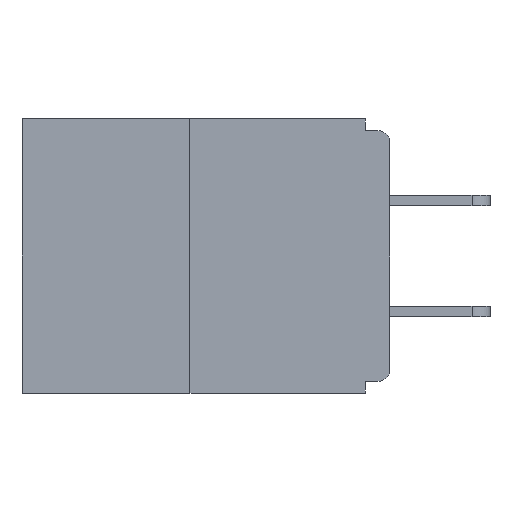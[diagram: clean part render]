
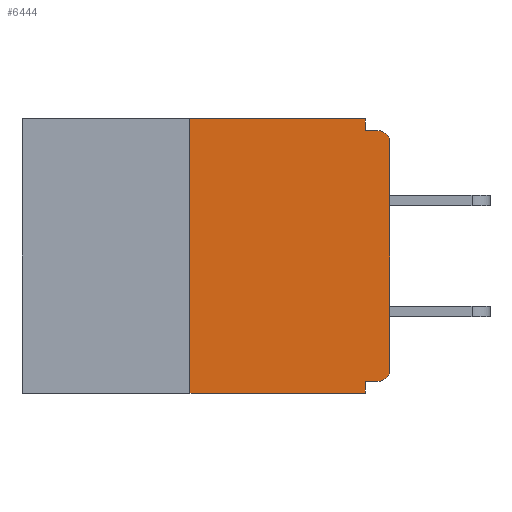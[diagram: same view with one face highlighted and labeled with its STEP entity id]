
A CAD part, left-side view. The second image highlights one B-rep face of the part: STEP entity #6444.
In plain terms, the highlighted planar face has unit normal (-1, 0, 0).
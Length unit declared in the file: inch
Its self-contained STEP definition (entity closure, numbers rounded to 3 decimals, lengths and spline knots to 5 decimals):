
#182 = VERTEX_POINT ( 'NONE', #7710 ) ;
#297 = ORIENTED_EDGE ( 'NONE', *, *, #10551, .T. ) ;
#424 = DIRECTION ( 'NONE',  ( 0., 1., 0. ) ) ;
#600 = ORIENTED_EDGE ( 'NONE', *, *, #10276, .T. ) ;
#846 = EDGE_CURVE ( 'NONE', #17180, #11150, #14406, .T. ) ;
#995 = LINE ( 'NONE', #12492, #16593 ) ;
#1286 = CARTESIAN_POINT ( 'NONE',  ( 0., 0.031, -0.015 ) ) ;
#1500 = CARTESIAN_POINT ( 'NONE',  ( 0., 0.031, -0.343 ) ) ;
#1552 = DIRECTION ( 'NONE',  ( 0., 0., 1. ) ) ;
#1807 = ORIENTED_EDGE ( 'NONE', *, *, #14363, .T. ) ;
#1910 = VECTOR ( 'NONE', #12389, 39.37008 ) ;
#2256 = CARTESIAN_POINT ( 'NONE',  ( 0., 0.031, -0.343 ) ) ;
#2279 = DIRECTION ( 'NONE',  ( 0., 0., -1. ) ) ;
#2557 = VECTOR ( 'NONE', #3654, 39.37008 ) ;
#3417 = ORIENTED_EDGE ( 'NONE', *, *, #14529, .F. ) ;
#3524 = LINE ( 'NONE', #6114, #14018 ) ;
#3570 = ORIENTED_EDGE ( 'NONE', *, *, #10451, .F. ) ;
#3654 = DIRECTION ( 'NONE',  ( 0., -1., 0. ) ) ;
#3727 = DIRECTION ( 'NONE',  ( 0., 0., 1. ) ) ;
#3900 = DIRECTION ( 'NONE',  ( 0., 0., -1. ) ) ;
#3932 = EDGE_CURVE ( 'NONE', #16206, #17180, #12841, .T. ) ;
#3948 = VERTEX_POINT ( 'NONE', #15938 ) ;
#3962 = PLANE ( 'NONE',  #10480 ) ;
#4166 = FACE_OUTER_BOUND ( 'NONE', #7609, .T. ) ;
#4472 = AXIS2_PLACEMENT_3D ( 'NONE', #9068, #15980, #2279 ) ;
#4695 = VERTEX_POINT ( 'NONE', #12079 ) ;
#5044 = CARTESIAN_POINT ( 'NONE',  ( 0., 0.25, 0. ) ) ;
#5382 = CARTESIAN_POINT ( 'NONE',  ( 0., 0.015, -0.328 ) ) ;
#5787 = EDGE_CURVE ( 'NONE', #13504, #9596, #6554, .T. ) ;
#6114 = CARTESIAN_POINT ( 'NONE',  ( 0., 0., -0.015 ) ) ;
#6289 = AXIS2_PLACEMENT_3D ( 'NONE', #17013, #10186, #7740 ) ;
#6444 = ADVANCED_FACE ( 'NONE', ( #4166 ), #3962, .F. ) ;
#6542 = VECTOR ( 'NONE', #424, 39.37008 ) ;
#6547 = ORIENTED_EDGE ( 'NONE', *, *, #5787, .T. ) ;
#6554 = LINE ( 'NONE', #6961, #10618 ) ;
#6961 = CARTESIAN_POINT ( 'NONE',  ( 0., 0.46, -0.343 ) ) ;
#6997 = CIRCLE ( 'NONE', #4472, 0.015 ) ;
#7045 = VECTOR ( 'NONE', #3727, 39.37008 ) ;
#7468 = LINE ( 'NONE', #5044, #7045 ) ;
#7609 = EDGE_LOOP ( 'NONE', ( #11813, #13123, #6547, #3417, #15741, #1807, #297, #600, #3570, #8094 ) ) ;
#7710 = CARTESIAN_POINT ( 'NONE',  ( 0., 0., -0.313 ) ) ;
#7727 = CIRCLE ( 'NONE', #6289, 0.015 ) ;
#7740 = DIRECTION ( 'NONE',  ( 0., 0., -1. ) ) ;
#8094 = ORIENTED_EDGE ( 'NONE', *, *, #846, .F. ) ;
#8153 = VERTEX_POINT ( 'NONE', #5382 ) ;
#8978 = CARTESIAN_POINT ( 'NONE',  ( 0., 0., -0.03 ) ) ;
#9068 = CARTESIAN_POINT ( 'NONE',  ( 0., 0.015, -0.03 ) ) ;
#9596 = VERTEX_POINT ( 'NONE', #2256 ) ;
#9600 = DIRECTION ( 'NONE',  ( 0., 0., -1. ) ) ;
#9666 = CARTESIAN_POINT ( 'NONE',  ( 0., 0.25, 0. ) ) ;
#10186 = DIRECTION ( 'NONE',  ( -1., 0., 0. ) ) ;
#10276 = EDGE_CURVE ( 'NONE', #13741, #3948, #6997, .T. ) ;
#10451 = EDGE_CURVE ( 'NONE', #11150, #3948, #3524, .T. ) ;
#10480 = AXIS2_PLACEMENT_3D ( 'NONE', #10918, #12302, #3900 ) ;
#10551 = EDGE_CURVE ( 'NONE', #182, #13741, #995, .T. ) ;
#10576 = CARTESIAN_POINT ( 'NONE',  ( 0., 0.25, -0.343 ) ) ;
#10618 = VECTOR ( 'NONE', #15252, 39.37008 ) ;
#10713 = EDGE_CURVE ( 'NONE', #8153, #4695, #11455, .T. ) ;
#10917 = LINE ( 'NONE', #1500, #1910 ) ;
#10918 = CARTESIAN_POINT ( 'NONE',  ( 0., 0.46, 0. ) ) ;
#11150 = VERTEX_POINT ( 'NONE', #1286 ) ;
#11455 = LINE ( 'NONE', #12730, #6542 ) ;
#11789 = CARTESIAN_POINT ( 'NONE',  ( 0., 0.031, 0. ) ) ;
#11813 = ORIENTED_EDGE ( 'NONE', *, *, #3932, .F. ) ;
#12079 = CARTESIAN_POINT ( 'NONE',  ( 0., 0.031, -0.328 ) ) ;
#12302 = DIRECTION ( 'NONE',  ( 1., 0., 0. ) ) ;
#12389 = DIRECTION ( 'NONE',  ( 0., 0., -1. ) ) ;
#12492 = CARTESIAN_POINT ( 'NONE',  ( 0., 0., 0. ) ) ;
#12730 = CARTESIAN_POINT ( 'NONE',  ( 0., 0., -0.328 ) ) ;
#12841 = LINE ( 'NONE', #13369, #2557 ) ;
#12978 = DIRECTION ( 'NONE',  ( 0., -1., 0. ) ) ;
#13123 = ORIENTED_EDGE ( 'NONE', *, *, #15565, .F. ) ;
#13369 = CARTESIAN_POINT ( 'NONE',  ( 0., 0.46, 0. ) ) ;
#13504 = VERTEX_POINT ( 'NONE', #10576 ) ;
#13741 = VERTEX_POINT ( 'NONE', #8978 ) ;
#14018 = VECTOR ( 'NONE', #12978, 39.37008 ) ;
#14363 = EDGE_CURVE ( 'NONE', #8153, #182, #7727, .T. ) ;
#14406 = LINE ( 'NONE', #14601, #15705 ) ;
#14529 = EDGE_CURVE ( 'NONE', #4695, #9596, #10917, .T. ) ;
#14601 = CARTESIAN_POINT ( 'NONE',  ( 0., 0.031, 0. ) ) ;
#15252 = DIRECTION ( 'NONE',  ( 0., -1., 0. ) ) ;
#15565 = EDGE_CURVE ( 'NONE', #13504, #16206, #7468, .T. ) ;
#15705 = VECTOR ( 'NONE', #9600, 39.37008 ) ;
#15741 = ORIENTED_EDGE ( 'NONE', *, *, #10713, .F. ) ;
#15938 = CARTESIAN_POINT ( 'NONE',  ( 0., 0.015, -0.015 ) ) ;
#15980 = DIRECTION ( 'NONE',  ( -1., 0., 0. ) ) ;
#16206 = VERTEX_POINT ( 'NONE', #9666 ) ;
#16593 = VECTOR ( 'NONE', #1552, 39.37008 ) ;
#17013 = CARTESIAN_POINT ( 'NONE',  ( 0., 0.015, -0.313 ) ) ;
#17180 = VERTEX_POINT ( 'NONE', #11789 ) ;
